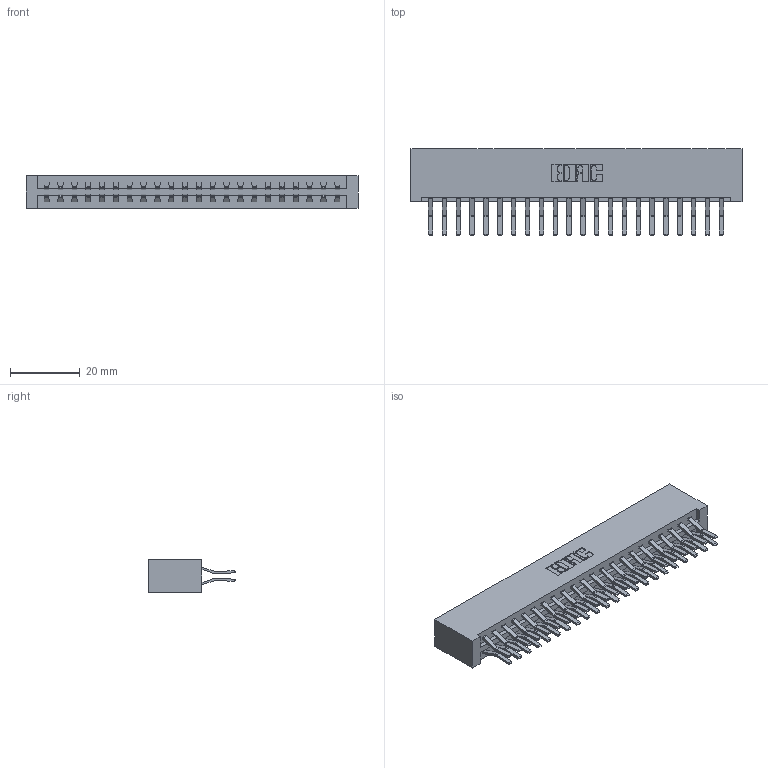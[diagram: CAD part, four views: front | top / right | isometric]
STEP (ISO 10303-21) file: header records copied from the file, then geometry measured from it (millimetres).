
FILE_DESCRIPTION (( 'STEP AP203' ), '1' );
FILE_NAME ('337-044-560-201.STEP', '2019-10-09T13:28:47', ( '' ), ( '' ), 'SwSTEP 2.0', 'SolidWorks 2016', '' );
FILE_SCHEMA (( 'CONFIG_CONTROL_DESIGN' ));
Length unit declared in the file: inch
Products named in the file (3): 345-292-001_560 Tail; 337 Part_No Mounting Lugs; 337-044-560-201
Assembly tree (45 placements, depth 2):
  337-044-560-201
    337 Part_No Mounting Lugs
    345-292-001_560 Tail  x44
Bounding box: 95.05 x 24.78 x 9.4 mm (x, y, z)
Volume: 10799.7 mm3; surface area: 12905.6 mm2
Topology: 45 solids, 45 shells, 2570 faces, 7635 edges, 5030 vertices
Faces by surface type: plane 1738, cylinder 832
Entity records: 19455 total; most frequent: CARTESIAN_POINT 3294, ORIENTED_EDGE 3230, DIRECTION 2835, EDGE_CURVE 1615, LINE 1491, VECTOR 1491, VERTEX_POINT 1074, AXIS2_PLACEMENT_3D 672
